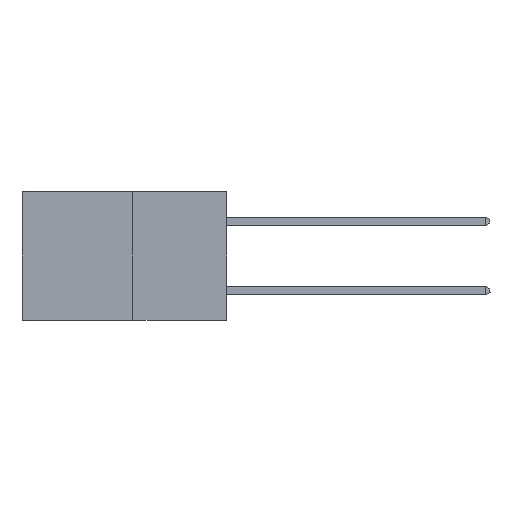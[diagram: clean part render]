
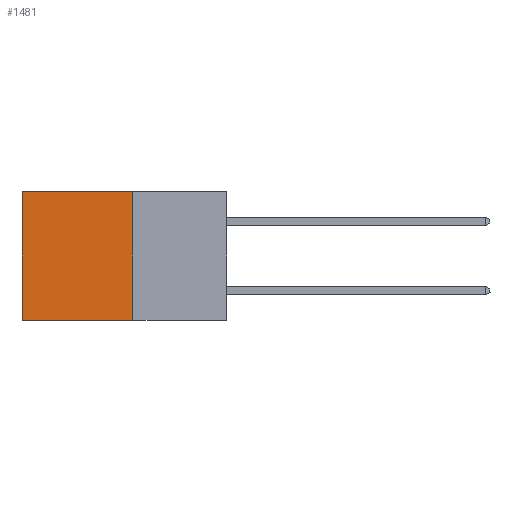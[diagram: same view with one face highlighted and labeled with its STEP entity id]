
A CAD part, left-side view. The second image highlights one B-rep face of the part: STEP entity #1481.
In plain terms, the highlighted planar face has unit normal (-1, 0, 0).
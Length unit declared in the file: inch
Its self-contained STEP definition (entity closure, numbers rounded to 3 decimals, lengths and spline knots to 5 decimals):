
#372 = EDGE_CURVE ( 'NONE', #1973, #8171, #4420, .T. ) ;
#419 = DIRECTION ( 'NONE',  ( 0., 0., -1. ) ) ;
#1481 = ADVANCED_FACE ( 'NONE', ( #5808 ), #6523, .F. ) ;
#1568 = CARTESIAN_POINT ( 'NONE',  ( 0.277, 0.59, 0. ) ) ;
#1816 = EDGE_CURVE ( 'NONE', #7630, #2272, #6073, .T. ) ;
#1876 = LINE ( 'NONE', #7051, #10649 ) ;
#1938 = EDGE_LOOP ( 'NONE', ( #8154, #2317, #2291, #5316 ) ) ;
#1973 = VERTEX_POINT ( 'NONE', #8325 ) ;
#2272 = VERTEX_POINT ( 'NONE', #4925 ) ;
#2291 = ORIENTED_EDGE ( 'NONE', *, *, #372, .F. ) ;
#2317 = ORIENTED_EDGE ( 'NONE', *, *, #3599, .F. ) ;
#2507 = DIRECTION ( 'NONE',  ( 1., 0., 0. ) ) ;
#2584 = DIRECTION ( 'NONE',  ( 0., 1., 0. ) ) ;
#3599 = EDGE_CURVE ( 'NONE', #8171, #2272, #6282, .T. ) ;
#4388 = DIRECTION ( 'NONE',  ( 0., 0., -1. ) ) ;
#4420 = LINE ( 'NONE', #10080, #8706 ) ;
#4925 = CARTESIAN_POINT ( 'NONE',  ( 0.277, 0.59, -0.37 ) ) ;
#5316 = ORIENTED_EDGE ( 'NONE', *, *, #9709, .T. ) ;
#5568 = DIRECTION ( 'NONE',  ( 0., 0., -1. ) ) ;
#5788 = CARTESIAN_POINT ( 'NONE',  ( 0.277, 0.27, -0.37 ) ) ;
#5808 = FACE_OUTER_BOUND ( 'NONE', #1938, .T. ) ;
#5874 = CARTESIAN_POINT ( 'NONE',  ( 0.277, 0.59, -0.37 ) ) ;
#6073 = LINE ( 'NONE', #5874, #10210 ) ;
#6282 = LINE ( 'NONE', #7130, #7972 ) ;
#6523 = PLANE ( 'NONE',  #7313 ) ;
#7020 = DIRECTION ( 'NONE',  ( 0., 1., 0. ) ) ;
#7051 = CARTESIAN_POINT ( 'NONE',  ( 0.277, 0.27, 0. ) ) ;
#7130 = CARTESIAN_POINT ( 'NONE',  ( 0.277, 0.27, -0.37 ) ) ;
#7313 = AXIS2_PLACEMENT_3D ( 'NONE', #5788, #2507, #419 ) ;
#7630 = VERTEX_POINT ( 'NONE', #1568 ) ;
#7972 = VECTOR ( 'NONE', #7020, 39.37008 ) ;
#8154 = ORIENTED_EDGE ( 'NONE', *, *, #1816, .T. ) ;
#8171 = VERTEX_POINT ( 'NONE', #10823 ) ;
#8325 = CARTESIAN_POINT ( 'NONE',  ( 0.277, 0.27, 0. ) ) ;
#8706 = VECTOR ( 'NONE', #4388, 39.37008 ) ;
#9709 = EDGE_CURVE ( 'NONE', #1973, #7630, #1876, .T. ) ;
#10080 = CARTESIAN_POINT ( 'NONE',  ( 0.277, 0.27, -0.37 ) ) ;
#10210 = VECTOR ( 'NONE', #5568, 39.37008 ) ;
#10649 = VECTOR ( 'NONE', #2584, 39.37008 ) ;
#10823 = CARTESIAN_POINT ( 'NONE',  ( 0.277, 0.27, -0.37 ) ) ;
